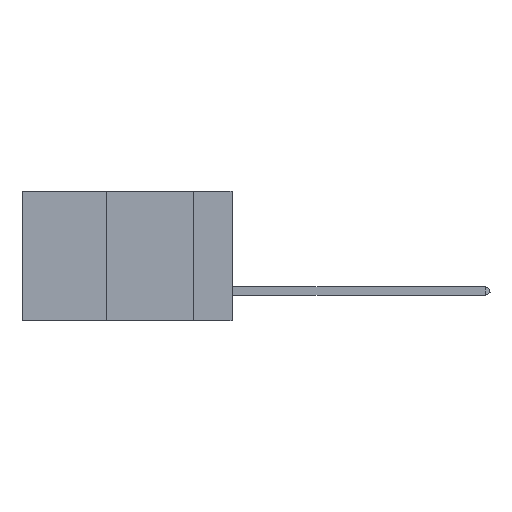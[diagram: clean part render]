
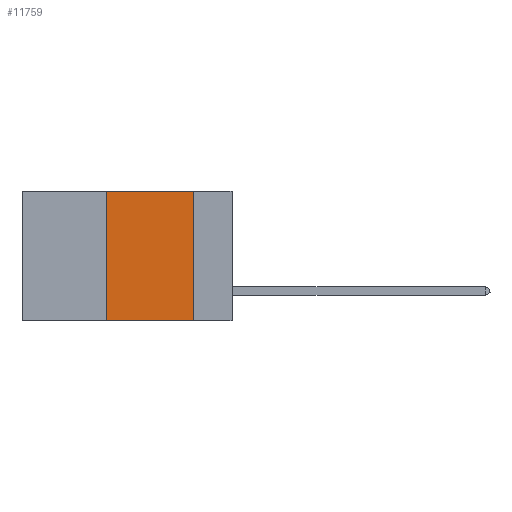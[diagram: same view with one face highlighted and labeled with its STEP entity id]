
A CAD part, left-side view. The second image highlights one B-rep face of the part: STEP entity #11759.
In plain terms, the highlighted planar face has unit normal (-1, 0, 0).
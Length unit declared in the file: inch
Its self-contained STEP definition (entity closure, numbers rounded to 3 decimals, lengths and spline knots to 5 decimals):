
#21 = DIRECTION ( 'NONE',  ( 0., 0., 1. ) ) ;
#1318 = EDGE_LOOP ( 'NONE', ( #14774, #9104, #10952, #9906 ) ) ;
#2065 = CARTESIAN_POINT ( 'NONE',  ( 0., 0.11, 0. ) ) ;
#2376 = DIRECTION ( 'NONE',  ( 0., -1., 0. ) ) ;
#2530 = LINE ( 'NONE', #14660, #12779 ) ;
#3440 = VERTEX_POINT ( 'NONE', #2065 ) ;
#3490 = CARTESIAN_POINT ( 'NONE',  ( 0., 0.36, 0. ) ) ;
#3601 = DIRECTION ( 'NONE',  ( 0., 0., -1. ) ) ;
#3655 = CARTESIAN_POINT ( 'NONE',  ( 0., 0.6, 0. ) ) ;
#5957 = PLANE ( 'NONE',  #12492 ) ;
#6209 = CARTESIAN_POINT ( 'NONE',  ( 0., 0.6, 0. ) ) ;
#6251 = VECTOR ( 'NONE', #2376, 39.37008 ) ;
#6394 = VERTEX_POINT ( 'NONE', #7322 ) ;
#6406 = EDGE_CURVE ( 'NONE', #3440, #12438, #2530, .T. ) ;
#6584 = EDGE_CURVE ( 'NONE', #6394, #12438, #14381, .T. ) ;
#7155 = EDGE_CURVE ( 'NONE', #12269, #3440, #10588, .T. ) ;
#7248 = VECTOR ( 'NONE', #11404, 39.37008 ) ;
#7322 = CARTESIAN_POINT ( 'NONE',  ( 0., 0.36, -0.37 ) ) ;
#8232 = EDGE_CURVE ( 'NONE', #6394, #12269, #12350, .T. ) ;
#8799 = CARTESIAN_POINT ( 'NONE',  ( 0., 0.6, -0.37 ) ) ;
#9104 = ORIENTED_EDGE ( 'NONE', *, *, #7155, .F. ) ;
#9405 = DIRECTION ( 'NONE',  ( 0., 0., -1. ) ) ;
#9906 = ORIENTED_EDGE ( 'NONE', *, *, #6584, .T. ) ;
#10588 = LINE ( 'NONE', #6209, #7248 ) ;
#10952 = ORIENTED_EDGE ( 'NONE', *, *, #8232, .F. ) ;
#11140 = FACE_OUTER_BOUND ( 'NONE', #1318, .T. ) ;
#11404 = DIRECTION ( 'NONE',  ( 0., -1., 0. ) ) ;
#11759 = ADVANCED_FACE ( 'NONE', ( #11140 ), #5957, .F. ) ;
#12036 = CARTESIAN_POINT ( 'NONE',  ( 0., 0.11, -0.37 ) ) ;
#12269 = VERTEX_POINT ( 'NONE', #3490 ) ;
#12350 = LINE ( 'NONE', #13649, #15332 ) ;
#12438 = VERTEX_POINT ( 'NONE', #12036 ) ;
#12492 = AXIS2_PLACEMENT_3D ( 'NONE', #3655, #13684, #3601 ) ;
#12779 = VECTOR ( 'NONE', #9405, 39.37008 ) ;
#13649 = CARTESIAN_POINT ( 'NONE',  ( 0., 0.36, 0. ) ) ;
#13684 = DIRECTION ( 'NONE',  ( 1., 0., 0. ) ) ;
#14381 = LINE ( 'NONE', #8799, #6251 ) ;
#14660 = CARTESIAN_POINT ( 'NONE',  ( 0., 0.11, 0. ) ) ;
#14774 = ORIENTED_EDGE ( 'NONE', *, *, #6406, .F. ) ;
#15332 = VECTOR ( 'NONE', #21, 39.37008 ) ;
